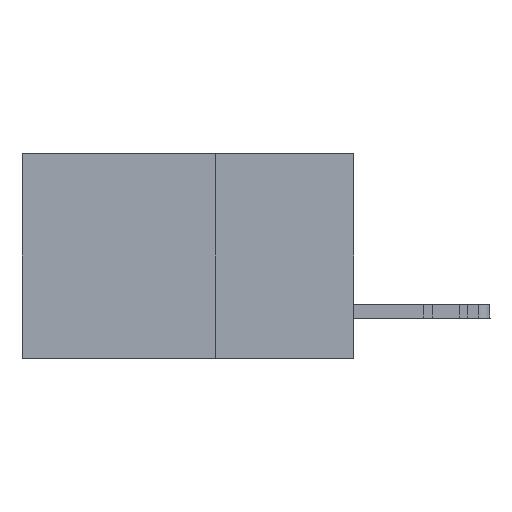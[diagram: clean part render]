
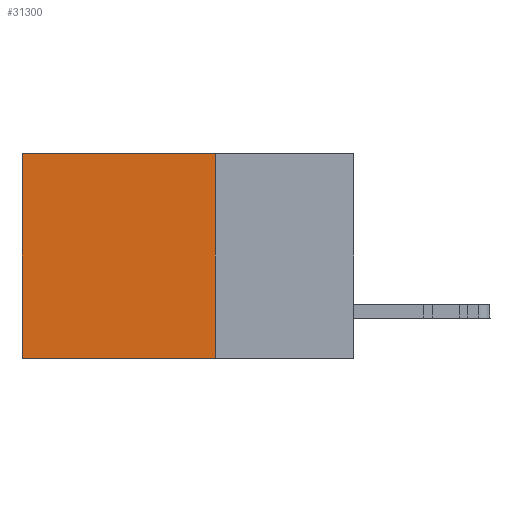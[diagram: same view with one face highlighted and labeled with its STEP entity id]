
A CAD part, left-side view. The second image highlights one B-rep face of the part: STEP entity #31300.
In plain terms, the highlighted planar face has unit normal (-1, 0, 0).
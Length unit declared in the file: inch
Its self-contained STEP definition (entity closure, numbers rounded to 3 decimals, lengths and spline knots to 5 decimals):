
#1477 = VECTOR ( 'NONE', #35195, 39.37008 ) ;
#2325 = PLANE ( 'NONE',  #16459 ) ;
#3744 = EDGE_CURVE ( 'NONE', #25753, #8879, #30382, .T. ) ;
#5526 = CARTESIAN_POINT ( 'NONE',  ( 0.2875, 0.25, -0.37 ) ) ;
#8879 = VERTEX_POINT ( 'NONE', #29877 ) ;
#9379 = LINE ( 'NONE', #5526, #19525 ) ;
#9971 = CARTESIAN_POINT ( 'NONE',  ( 0.2875, 0.25, 0. ) ) ;
#10926 = EDGE_CURVE ( 'NONE', #25753, #14744, #41959, .T. ) ;
#11087 = CARTESIAN_POINT ( 'NONE',  ( 0.2875, 0.25, 0. ) ) ;
#11601 = CARTESIAN_POINT ( 'NONE',  ( 0.2875, 0.6, -0.37 ) ) ;
#12359 = VECTOR ( 'NONE', #33305, 39.37008 ) ;
#14744 = VERTEX_POINT ( 'NONE', #17716 ) ;
#15668 = FACE_OUTER_BOUND ( 'NONE', #41650, .T. ) ;
#15950 = LINE ( 'NONE', #22497, #32035 ) ;
#16459 = AXIS2_PLACEMENT_3D ( 'NONE', #39541, #29426, #36148 ) ;
#17716 = CARTESIAN_POINT ( 'NONE',  ( 0.2875, 0.25, -0.37 ) ) ;
#19307 = ORIENTED_EDGE ( 'NONE', *, *, #10926, .F. ) ;
#19332 = DIRECTION ( 'NONE',  ( 0., 1., 0. ) ) ;
#19525 = VECTOR ( 'NONE', #19332, 39.37008 ) ;
#20727 = ORIENTED_EDGE ( 'NONE', *, *, #30977, .F. ) ;
#22497 = CARTESIAN_POINT ( 'NONE',  ( 0.2875, 0.6, 0. ) ) ;
#25648 = VERTEX_POINT ( 'NONE', #11601 ) ;
#25753 = VERTEX_POINT ( 'NONE', #9971 ) ;
#29426 = DIRECTION ( 'NONE',  ( 1., 0., 0. ) ) ;
#29705 = DIRECTION ( 'NONE',  ( 0., 0., -1. ) ) ;
#29877 = CARTESIAN_POINT ( 'NONE',  ( 0.2875, 0.6, 0. ) ) ;
#30382 = LINE ( 'NONE', #43854, #12359 ) ;
#30977 = EDGE_CURVE ( 'NONE', #14744, #25648, #9379, .T. ) ;
#31300 = ADVANCED_FACE ( 'NONE', ( #15668 ), #2325, .F. ) ;
#32035 = VECTOR ( 'NONE', #29705, 39.37008 ) ;
#33297 = ORIENTED_EDGE ( 'NONE', *, *, #42187, .T. ) ;
#33305 = DIRECTION ( 'NONE',  ( 0., 1., 0. ) ) ;
#35195 = DIRECTION ( 'NONE',  ( 0., 0., -1. ) ) ;
#36148 = DIRECTION ( 'NONE',  ( 0., 0., -1. ) ) ;
#39541 = CARTESIAN_POINT ( 'NONE',  ( 0.2875, 0.25, 0. ) ) ;
#39590 = ORIENTED_EDGE ( 'NONE', *, *, #3744, .T. ) ;
#41650 = EDGE_LOOP ( 'NONE', ( #33297, #20727, #19307, #39590 ) ) ;
#41959 = LINE ( 'NONE', #11087, #1477 ) ;
#42187 = EDGE_CURVE ( 'NONE', #8879, #25648, #15950, .T. ) ;
#43854 = CARTESIAN_POINT ( 'NONE',  ( 0.2875, 0.25, 0. ) ) ;
